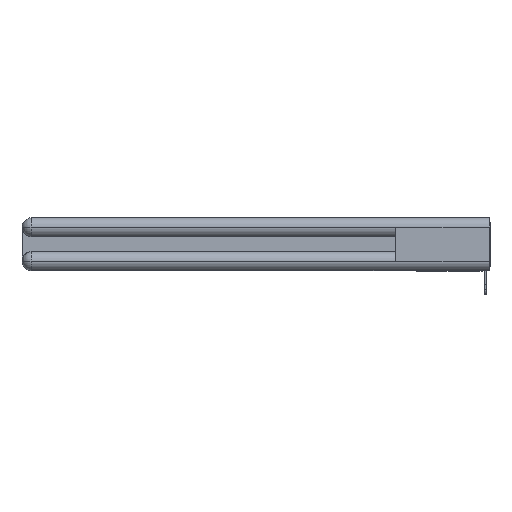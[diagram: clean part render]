
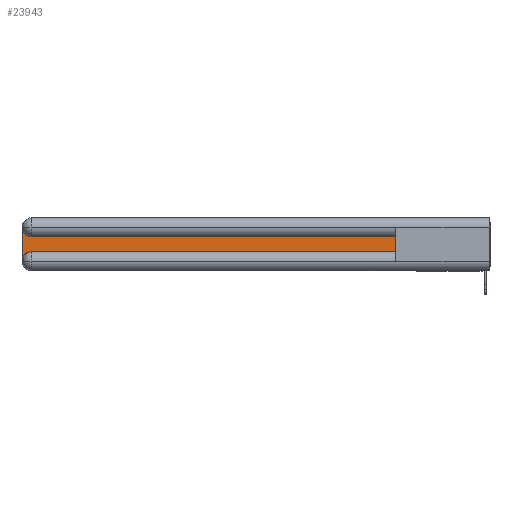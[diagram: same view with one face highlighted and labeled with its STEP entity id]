
A CAD part, left-side view. The second image highlights one B-rep face of the part: STEP entity #23943.
In plain terms, the highlighted planar face has unit normal (-1, 0, 0).
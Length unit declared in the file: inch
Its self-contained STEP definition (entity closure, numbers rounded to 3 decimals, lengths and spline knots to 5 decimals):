
#260 = DIRECTION ( 'NONE',  ( 1., 0., 0. ) ) ;
#1398 = CARTESIAN_POINT ( 'NONE',  ( 0.075, 3., -0.2775 ) ) ;
#1561 = LINE ( 'NONE', #18110, #22407 ) ;
#1823 = EDGE_CURVE ( 'NONE', #27286, #6152, #7112, .T. ) ;
#2738 = LINE ( 'NONE', #9577, #24971 ) ;
#3159 = ORIENTED_EDGE ( 'NONE', *, *, #26745, .T. ) ;
#3569 = AXIS2_PLACEMENT_3D ( 'NONE', #6328, #14790, #25430 ) ;
#4213 = AXIS2_PLACEMENT_3D ( 'NONE', #13108, #260, #17836 ) ;
#4663 = ORIENTED_EDGE ( 'NONE', *, *, #1823, .T. ) ;
#5403 = DIRECTION ( 'NONE',  ( 1., 0., 0. ) ) ;
#5834 = FACE_OUTER_BOUND ( 'NONE', #18294, .T. ) ;
#6152 = VERTEX_POINT ( 'NONE', #14508 ) ;
#6328 = CARTESIAN_POINT ( 'NONE',  ( 0.075, 2.94, -0.2775 ) ) ;
#7112 = CIRCLE ( 'NONE', #3569, 0.06 ) ;
#7900 = DIRECTION ( 'NONE',  ( 0., 0., 1. ) ) ;
#8233 = AXIS2_PLACEMENT_3D ( 'NONE', #9322, #5403, #22535 ) ;
#8303 = CARTESIAN_POINT ( 'NONE',  ( 0.075, 0.6, -0.1225 ) ) ;
#8608 = ORIENTED_EDGE ( 'NONE', *, *, #10247, .T. ) ;
#8660 = CIRCLE ( 'NONE', #8233, 0.06 ) ;
#9322 = CARTESIAN_POINT ( 'NONE',  ( 0.075, 2.94, -0.0625 ) ) ;
#9577 = CARTESIAN_POINT ( 'NONE',  ( 0.075, 0.6, -0.2175 ) ) ;
#10247 = EDGE_CURVE ( 'NONE', #17394, #13309, #8660, .T. ) ;
#11138 = VERTEX_POINT ( 'NONE', #8303 ) ;
#13108 = CARTESIAN_POINT ( 'NONE',  ( 0.075, 3., -0.1225 ) ) ;
#13309 = VERTEX_POINT ( 'NONE', #15008 ) ;
#13603 = VECTOR ( 'NONE', #7900, 39.37008 ) ;
#14137 = DIRECTION ( 'NONE',  ( 0., 0., -1. ) ) ;
#14269 = EDGE_CURVE ( 'NONE', #6152, #23360, #2738, .T. ) ;
#14508 = CARTESIAN_POINT ( 'NONE',  ( 0.075, 2.94, -0.2175 ) ) ;
#14790 = DIRECTION ( 'NONE',  ( 1., 0., 0. ) ) ;
#15008 = CARTESIAN_POINT ( 'NONE',  ( 0.075, 3., -0.0625 ) ) ;
#15656 = LINE ( 'NONE', #26840, #17375 ) ;
#15755 = DIRECTION ( 'NONE',  ( 0., 1., 0. ) ) ;
#17375 = VECTOR ( 'NONE', #14137, 39.37008 ) ;
#17394 = VERTEX_POINT ( 'NONE', #20721 ) ;
#17774 = EDGE_CURVE ( 'NONE', #11138, #17394, #1561, .T. ) ;
#17836 = DIRECTION ( 'NONE',  ( 0., 0., -1. ) ) ;
#18110 = CARTESIAN_POINT ( 'NONE',  ( 0.075, 0.6, -0.1225 ) ) ;
#18294 = EDGE_LOOP ( 'NONE', ( #21342, #8608, #18797, #4663, #23311, #3159 ) ) ;
#18797 = ORIENTED_EDGE ( 'NONE', *, *, #22405, .T. ) ;
#20721 = CARTESIAN_POINT ( 'NONE',  ( 0.075, 2.94, -0.1225 ) ) ;
#21342 = ORIENTED_EDGE ( 'NONE', *, *, #17774, .T. ) ;
#21421 = LINE ( 'NONE', #24927, #13603 ) ;
#22405 = EDGE_CURVE ( 'NONE', #13309, #27286, #15656, .T. ) ;
#22407 = VECTOR ( 'NONE', #15755, 39.37008 ) ;
#22535 = DIRECTION ( 'NONE',  ( 0., 0., -1. ) ) ;
#23311 = ORIENTED_EDGE ( 'NONE', *, *, #14269, .T. ) ;
#23360 = VERTEX_POINT ( 'NONE', #27845 ) ;
#23943 = ADVANCED_FACE ( 'NONE', ( #5834 ), #25741, .F. ) ;
#24927 = CARTESIAN_POINT ( 'NONE',  ( 0.075, 0.6, -0.2175 ) ) ;
#24971 = VECTOR ( 'NONE', #26989, 39.37008 ) ;
#25430 = DIRECTION ( 'NONE',  ( 0., 0., -1. ) ) ;
#25741 = PLANE ( 'NONE',  #4213 ) ;
#26745 = EDGE_CURVE ( 'NONE', #23360, #11138, #21421, .T. ) ;
#26840 = CARTESIAN_POINT ( 'NONE',  ( 0.075, 3., -0.2175 ) ) ;
#26989 = DIRECTION ( 'NONE',  ( 0., -1., 0. ) ) ;
#27286 = VERTEX_POINT ( 'NONE', #1398 ) ;
#27845 = CARTESIAN_POINT ( 'NONE',  ( 0.075, 0.6, -0.2175 ) ) ;
